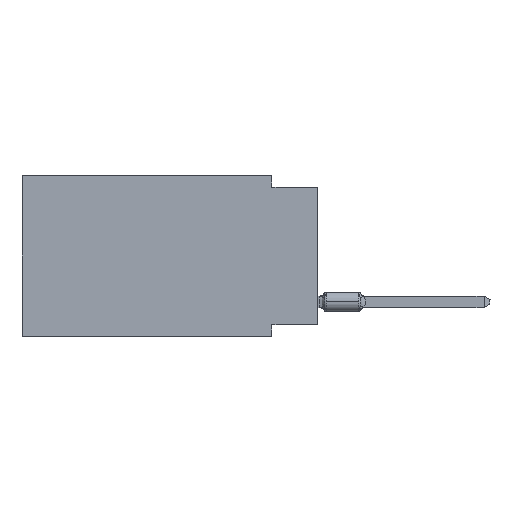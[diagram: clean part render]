
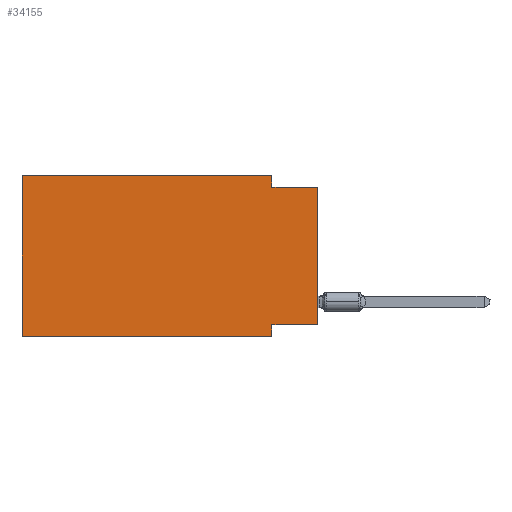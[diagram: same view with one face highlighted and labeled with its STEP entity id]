
A CAD part, left-side view. The second image highlights one B-rep face of the part: STEP entity #34155.
In plain terms, the highlighted planar face has unit normal (-1, 0, 0).
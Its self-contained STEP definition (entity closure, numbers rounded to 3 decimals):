
#386 = DIRECTION ( 'NONE',  ( 0., 1., 0. ) ) ;
#557 = CARTESIAN_POINT ( 'NONE',  ( 0., 0., -8.255 ) ) ;
#1612 = DIRECTION ( 'NONE',  ( 1., 0., 0. ) ) ;
#1642 = DIRECTION ( 'NONE',  ( 0., 0., -1. ) ) ;
#3057 = VECTOR ( 'NONE', #1642, 1000. ) ;
#3110 = VECTOR ( 'NONE', #10141, 1000. ) ;
#3306 = LINE ( 'NONE', #557, #24622 ) ;
#5138 = VERTEX_POINT ( 'NONE', #22463 ) ;
#5587 = EDGE_CURVE ( 'NONE', #22566, #10122, #19854, .T. ) ;
#6001 = CARTESIAN_POINT ( 'NONE',  ( 0., 0., -0.635 ) ) ;
#6942 = CARTESIAN_POINT ( 'NONE',  ( 0., 0., -8.255 ) ) ;
#6997 = ORIENTED_EDGE ( 'NONE', *, *, #35242, .F. ) ;
#7768 = CARTESIAN_POINT ( 'NONE',  ( 0., 0., 0. ) ) ;
#7966 = CARTESIAN_POINT ( 'NONE',  ( 0., 2.54, -8.89 ) ) ;
#8443 = CARTESIAN_POINT ( 'NONE',  ( 0., 16.383, -8.89 ) ) ;
#8846 = VECTOR ( 'NONE', #23781, 1000. ) ;
#9822 = VERTEX_POINT ( 'NONE', #33039 ) ;
#10122 = VERTEX_POINT ( 'NONE', #26988 ) ;
#10141 = DIRECTION ( 'NONE',  ( 0., -1., 0. ) ) ;
#10381 = LINE ( 'NONE', #31893, #3057 ) ;
#10640 = EDGE_CURVE ( 'NONE', #16413, #10122, #21077, .T. ) ;
#11240 = VERTEX_POINT ( 'NONE', #8443 ) ;
#11515 = EDGE_CURVE ( 'NONE', #11240, #9822, #24086, .T. ) ;
#12900 = PLANE ( 'NONE',  #21623 ) ;
#13086 = CARTESIAN_POINT ( 'NONE',  ( 0., 16.383, 0. ) ) ;
#14033 = VECTOR ( 'NONE', #17128, 1000. ) ;
#15509 = VECTOR ( 'NONE', #23992, 1000. ) ;
#16413 = VERTEX_POINT ( 'NONE', #6942 ) ;
#17128 = DIRECTION ( 'NONE',  ( 0., -1., 0. ) ) ;
#17575 = ORIENTED_EDGE ( 'NONE', *, *, #24108, .F. ) ;
#17800 = ORIENTED_EDGE ( 'NONE', *, *, #28873, .F. ) ;
#18131 = LINE ( 'NONE', #23968, #8846 ) ;
#19854 = LINE ( 'NONE', #6001, #14033 ) ;
#21077 = LINE ( 'NONE', #7768, #15509 ) ;
#21612 = CARTESIAN_POINT ( 'NONE',  ( 0., 16.383, 0. ) ) ;
#21623 = AXIS2_PLACEMENT_3D ( 'NONE', #13086, #1612, #24015 ) ;
#21793 = LINE ( 'NONE', #21612, #3110 ) ;
#22326 = LINE ( 'NONE', #28155, #24642 ) ;
#22463 = CARTESIAN_POINT ( 'NONE',  ( 0., 2.54, -8.255 ) ) ;
#22566 = VERTEX_POINT ( 'NONE', #25921 ) ;
#23781 = DIRECTION ( 'NONE',  ( 0., -1., 0. ) ) ;
#23870 = EDGE_CURVE ( 'NONE', #9822, #34914, #21793, .T. ) ;
#23968 = CARTESIAN_POINT ( 'NONE',  ( 0., 16.383, -8.89 ) ) ;
#23992 = DIRECTION ( 'NONE',  ( 0., 0., 1. ) ) ;
#24015 = DIRECTION ( 'NONE',  ( 0., 0., -1. ) ) ;
#24086 = LINE ( 'NONE', #31752, #35048 ) ;
#24108 = EDGE_CURVE ( 'NONE', #5138, #33031, #22326, .T. ) ;
#24328 = ORIENTED_EDGE ( 'NONE', *, *, #10640, .T. ) ;
#24622 = VECTOR ( 'NONE', #386, 1000. ) ;
#24642 = VECTOR ( 'NONE', #24881, 1000. ) ;
#24881 = DIRECTION ( 'NONE',  ( 0., 0., -1. ) ) ;
#25292 = ORIENTED_EDGE ( 'NONE', *, *, #34576, .T. ) ;
#25566 = EDGE_LOOP ( 'NONE', ( #24328, #32723, #6997, #35798, #28083, #25292, #17575, #17800 ) ) ;
#25921 = CARTESIAN_POINT ( 'NONE',  ( 0., 2.54, -0.635 ) ) ;
#26988 = CARTESIAN_POINT ( 'NONE',  ( 0., 0., -0.635 ) ) ;
#28083 = ORIENTED_EDGE ( 'NONE', *, *, #11515, .F. ) ;
#28155 = CARTESIAN_POINT ( 'NONE',  ( 0., 2.54, -8.89 ) ) ;
#28873 = EDGE_CURVE ( 'NONE', #16413, #5138, #3306, .T. ) ;
#29310 = FACE_OUTER_BOUND ( 'NONE', #25566, .T. ) ;
#31752 = CARTESIAN_POINT ( 'NONE',  ( 0., 16.383, 0. ) ) ;
#31893 = CARTESIAN_POINT ( 'NONE',  ( 0., 2.54, 0. ) ) ;
#32135 = CARTESIAN_POINT ( 'NONE',  ( 0., 2.54, 0. ) ) ;
#32723 = ORIENTED_EDGE ( 'NONE', *, *, #5587, .F. ) ;
#33031 = VERTEX_POINT ( 'NONE', #7966 ) ;
#33039 = CARTESIAN_POINT ( 'NONE',  ( 0., 16.383, 0. ) ) ;
#34155 = ADVANCED_FACE ( 'NONE', ( #29310 ), #12900, .F. ) ;
#34576 = EDGE_CURVE ( 'NONE', #11240, #33031, #18131, .T. ) ;
#34914 = VERTEX_POINT ( 'NONE', #32135 ) ;
#35048 = VECTOR ( 'NONE', #35208, 1000. ) ;
#35208 = DIRECTION ( 'NONE',  ( 0., 0., 1. ) ) ;
#35242 = EDGE_CURVE ( 'NONE', #34914, #22566, #10381, .T. ) ;
#35798 = ORIENTED_EDGE ( 'NONE', *, *, #23870, .F. ) ;
